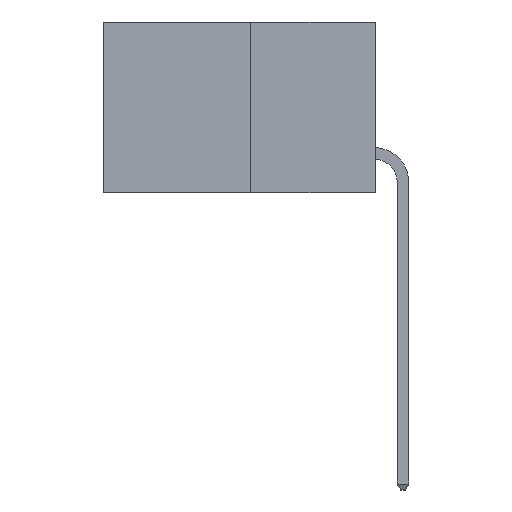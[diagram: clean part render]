
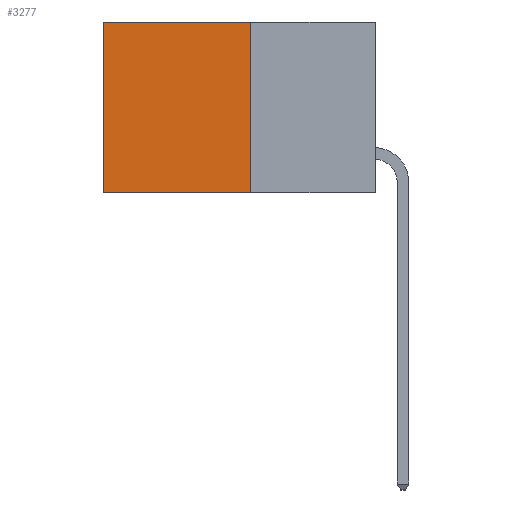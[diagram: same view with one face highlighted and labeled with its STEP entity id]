
A CAD part, left-side view. The second image highlights one B-rep face of the part: STEP entity #3277.
In plain terms, the highlighted planar face has unit normal (-1, 0, 0).
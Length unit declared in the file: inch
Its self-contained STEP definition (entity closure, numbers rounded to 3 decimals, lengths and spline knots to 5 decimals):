
#114 = DIRECTION ( 'NONE',  ( 0., 1., 0. ) ) ;
#131 = LINE ( 'NONE', #2329, #7292 ) ;
#297 = DIRECTION ( 'NONE',  ( 1., 0., 0. ) ) ;
#657 = VERTEX_POINT ( 'NONE', #6194 ) ;
#963 = PLANE ( 'NONE',  #1097 ) ;
#1097 = AXIS2_PLACEMENT_3D ( 'NONE', #3893, #297, #9727 ) ;
#1384 = CARTESIAN_POINT ( 'NONE',  ( 0.277, 0.27, -0.37 ) ) ;
#2079 = EDGE_CURVE ( 'NONE', #8392, #9264, #11329, .T. ) ;
#2309 = CARTESIAN_POINT ( 'NONE',  ( 0.277, 0.59, -0.37 ) ) ;
#2329 = CARTESIAN_POINT ( 'NONE',  ( 0.277, 0.27, 0. ) ) ;
#2372 = DIRECTION ( 'NONE',  ( 0., 0., -1. ) ) ;
#2691 = LINE ( 'NONE', #9463, #7407 ) ;
#3089 = EDGE_CURVE ( 'NONE', #657, #8329, #6416, .T. ) ;
#3184 = ORIENTED_EDGE ( 'NONE', *, *, #3089, .F. ) ;
#3237 = DIRECTION ( 'NONE',  ( 0., 1., 0. ) ) ;
#3277 = ADVANCED_FACE ( 'NONE', ( #9078 ), #963, .F. ) ;
#3582 = CARTESIAN_POINT ( 'NONE',  ( 0.277, 0.59, -0.37 ) ) ;
#3893 = CARTESIAN_POINT ( 'NONE',  ( 0.277, 0.27, -0.37 ) ) ;
#4632 = DIRECTION ( 'NONE',  ( 0., 0., -1. ) ) ;
#4637 = CARTESIAN_POINT ( 'NONE',  ( 0.277, 0.27, -0.37 ) ) ;
#5376 = ORIENTED_EDGE ( 'NONE', *, *, #7745, .T. ) ;
#6108 = CARTESIAN_POINT ( 'NONE',  ( 0.277, 0.59, 0. ) ) ;
#6194 = CARTESIAN_POINT ( 'NONE',  ( 0.277, 0.27, 0. ) ) ;
#6416 = LINE ( 'NONE', #4637, #11744 ) ;
#7292 = VECTOR ( 'NONE', #3237, 39.37008 ) ;
#7407 = VECTOR ( 'NONE', #114, 39.37008 ) ;
#7466 = ORIENTED_EDGE ( 'NONE', *, *, #8770, .F. ) ;
#7745 = EDGE_CURVE ( 'NONE', #657, #8392, #131, .T. ) ;
#7750 = EDGE_LOOP ( 'NONE', ( #8347, #7466, #3184, #5376 ) ) ;
#8329 = VERTEX_POINT ( 'NONE', #1384 ) ;
#8347 = ORIENTED_EDGE ( 'NONE', *, *, #2079, .T. ) ;
#8392 = VERTEX_POINT ( 'NONE', #6108 ) ;
#8770 = EDGE_CURVE ( 'NONE', #8329, #9264, #2691, .T. ) ;
#9078 = FACE_OUTER_BOUND ( 'NONE', #7750, .T. ) ;
#9264 = VERTEX_POINT ( 'NONE', #3582 ) ;
#9463 = CARTESIAN_POINT ( 'NONE',  ( 0.277, 0.27, -0.37 ) ) ;
#9727 = DIRECTION ( 'NONE',  ( 0., 0., -1. ) ) ;
#11031 = VECTOR ( 'NONE', #4632, 39.37008 ) ;
#11329 = LINE ( 'NONE', #2309, #11031 ) ;
#11744 = VECTOR ( 'NONE', #2372, 39.37008 ) ;
